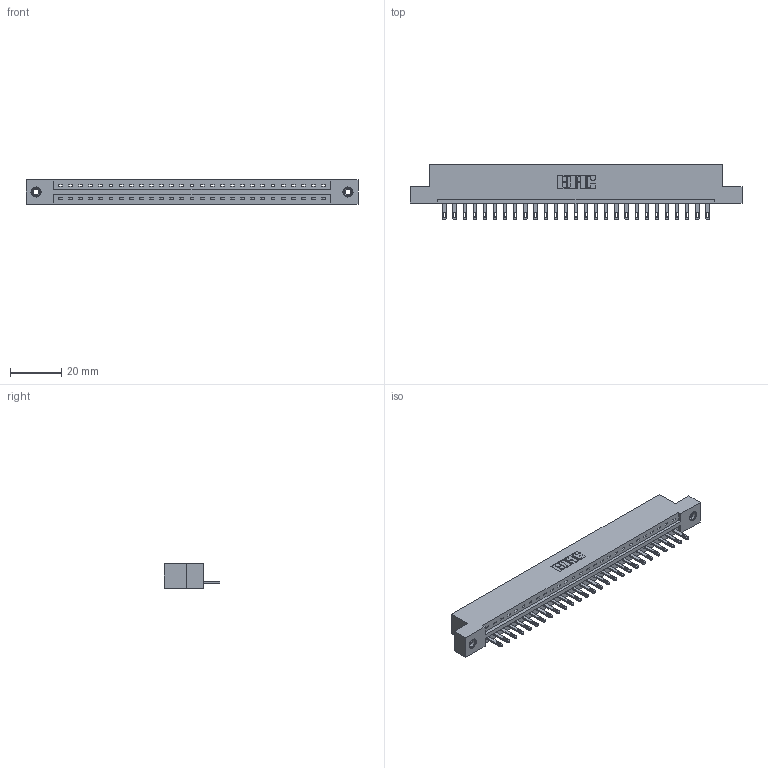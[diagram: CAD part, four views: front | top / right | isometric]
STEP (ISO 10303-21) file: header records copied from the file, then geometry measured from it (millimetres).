
FILE_DESCRIPTION (( 'STEP AP203' ), '1' );
FILE_NAME ('337-027-500-108.STEP', '2019-09-30T19:14:30', ( '' ), ( '' ), 'SwSTEP 2.0', 'SolidWorks 2016', '' );
FILE_SCHEMA (( 'CONFIG_CONTROL_DESIGN' ));
Length unit declared in the file: inch
Products named in the file (4): 345-250-001_345-250-003-102; 337 Part_Flush Mounting Lugs - 0.156 Dia-TI; 345-292-001_345-293-100; 337-027-500-108
Assembly tree (30 placements, depth 2):
  337-027-500-108
    337 Part_Flush Mounting Lugs - 0.156 Dia-TI
    345-292-001_345-293-100  x27
    345-250-001_345-250-003-102  x2
Bounding box: 130 x 21.85 x 9.4 mm (x, y, z)
Volume: 13333.5 mm3; surface area: 13787.7 mm2
Topology: 30 solids, 30 shells, 1740 faces, 5307 edges, 3530 vertices
Faces by surface type: plane 1182, cylinder 542, cone 12, torus 4
Entity records: 23126 total; most frequent: CARTESIAN_POINT 4006, ORIENTED_EDGE 3962, DIRECTION 3437, EDGE_CURVE 1981, LINE 1829, VECTOR 1829, VERTEX_POINT 1316, AXIS2_PLACEMENT_3D 804
